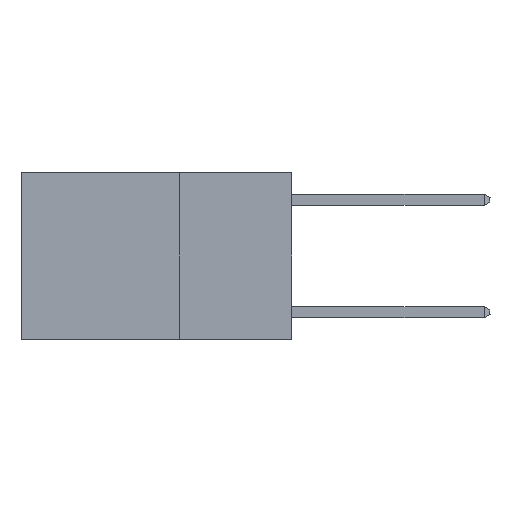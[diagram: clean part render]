
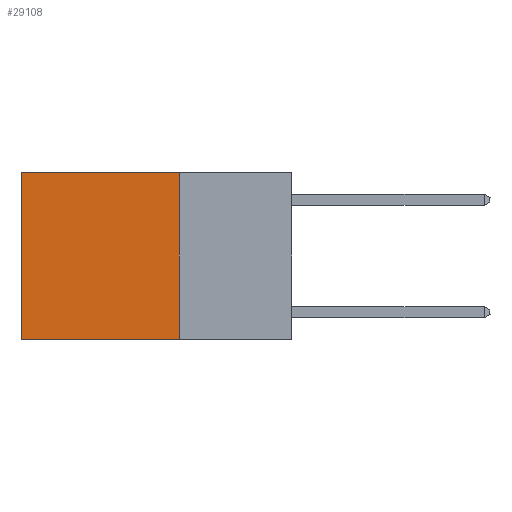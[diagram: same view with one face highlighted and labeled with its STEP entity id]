
A CAD part, left-side view. The second image highlights one B-rep face of the part: STEP entity #29108.
In plain terms, the highlighted planar face has unit normal (-1, 0, 0).
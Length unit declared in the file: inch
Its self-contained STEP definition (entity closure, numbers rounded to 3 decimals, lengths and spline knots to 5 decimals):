
#2262 = AXIS2_PLACEMENT_3D ( 'NONE', #8763, #12117, #24653 ) ;
#2523 = ORIENTED_EDGE ( 'NONE', *, *, #15830, .T. ) ;
#5278 = ORIENTED_EDGE ( 'NONE', *, *, #8709, .F. ) ;
#5968 = VERTEX_POINT ( 'NONE', #17026 ) ;
#7515 = CARTESIAN_POINT ( 'NONE',  ( 0.2625, 0.6, 0. ) ) ;
#8709 = EDGE_CURVE ( 'NONE', #11571, #5968, #16766, .T. ) ;
#8763 = CARTESIAN_POINT ( 'NONE',  ( 0.2625, 0.25, 0. ) ) ;
#8860 = VECTOR ( 'NONE', #14886, 39.37008 ) ;
#9677 = CARTESIAN_POINT ( 'NONE',  ( 0.2625, 0.25, -0.37 ) ) ;
#9918 = LINE ( 'NONE', #7515, #8860 ) ;
#10088 = VECTOR ( 'NONE', #29008, 39.37008 ) ;
#11171 = PLANE ( 'NONE',  #2262 ) ;
#11571 = VERTEX_POINT ( 'NONE', #28517 ) ;
#12117 = DIRECTION ( 'NONE',  ( 1., 0., 0. ) ) ;
#13576 = FACE_OUTER_BOUND ( 'NONE', #28478, .T. ) ;
#13612 = EDGE_CURVE ( 'NONE', #31384, #24147, #30585, .T. ) ;
#14322 = DIRECTION ( 'NONE',  ( 0., 0., -1. ) ) ;
#14641 = CARTESIAN_POINT ( 'NONE',  ( 0.2625, 0.25, 0. ) ) ;
#14886 = DIRECTION ( 'NONE',  ( 0., 0., -1. ) ) ;
#15830 = EDGE_CURVE ( 'NONE', #24147, #5968, #9918, .T. ) ;
#16766 = LINE ( 'NONE', #9677, #10088 ) ;
#17026 = CARTESIAN_POINT ( 'NONE',  ( 0.2625, 0.6, -0.37 ) ) ;
#17775 = CARTESIAN_POINT ( 'NONE',  ( 0.2625, 0.6, 0. ) ) ;
#18656 = CARTESIAN_POINT ( 'NONE',  ( 0.2625, 0.25, 0. ) ) ;
#19639 = ORIENTED_EDGE ( 'NONE', *, *, #21514, .F. ) ;
#19668 = VECTOR ( 'NONE', #28480, 39.37008 ) ;
#19911 = VECTOR ( 'NONE', #14322, 39.37008 ) ;
#21514 = EDGE_CURVE ( 'NONE', #31384, #11571, #29001, .T. ) ;
#23570 = CARTESIAN_POINT ( 'NONE',  ( 0.2625, 0.25, 0. ) ) ;
#24147 = VERTEX_POINT ( 'NONE', #17775 ) ;
#24653 = DIRECTION ( 'NONE',  ( 0., 0., -1. ) ) ;
#28478 = EDGE_LOOP ( 'NONE', ( #2523, #5278, #19639, #30819 ) ) ;
#28480 = DIRECTION ( 'NONE',  ( 0., 1., 0. ) ) ;
#28517 = CARTESIAN_POINT ( 'NONE',  ( 0.2625, 0.25, -0.37 ) ) ;
#29001 = LINE ( 'NONE', #14641, #19911 ) ;
#29008 = DIRECTION ( 'NONE',  ( 0., 1., 0. ) ) ;
#29108 = ADVANCED_FACE ( 'NONE', ( #13576 ), #11171, .F. ) ;
#30585 = LINE ( 'NONE', #18656, #19668 ) ;
#30819 = ORIENTED_EDGE ( 'NONE', *, *, #13612, .T. ) ;
#31384 = VERTEX_POINT ( 'NONE', #23570 ) ;
